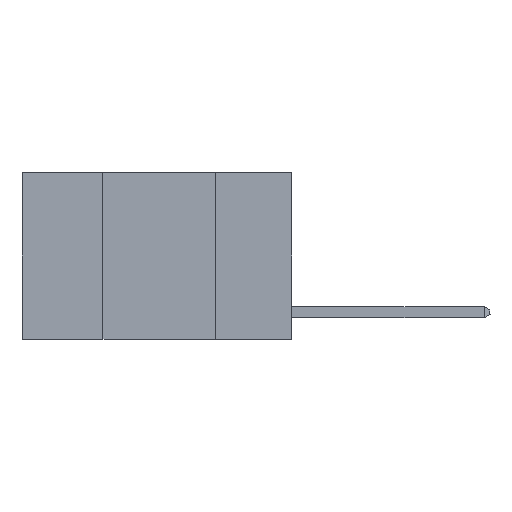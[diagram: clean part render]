
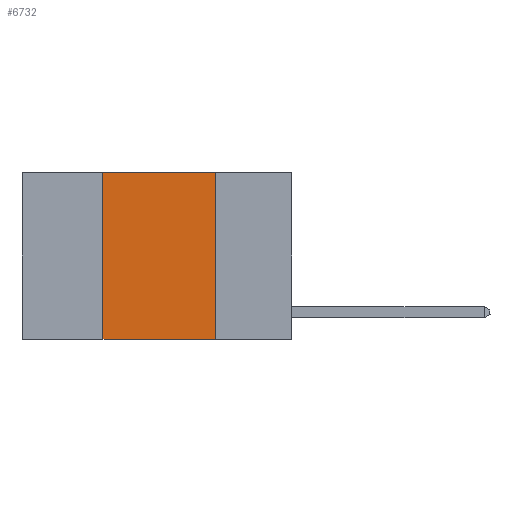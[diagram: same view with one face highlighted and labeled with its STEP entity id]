
A CAD part, left-side view. The second image highlights one B-rep face of the part: STEP entity #6732.
In plain terms, the highlighted planar face has unit normal (-1, 0, 0).
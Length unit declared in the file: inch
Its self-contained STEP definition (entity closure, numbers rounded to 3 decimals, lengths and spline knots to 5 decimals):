
#153 = EDGE_CURVE ( 'NONE', #2422, #431, #4611, .T. ) ;
#431 = VERTEX_POINT ( 'NONE', #10869 ) ;
#643 = VECTOR ( 'NONE', #11021, 39.37008 ) ;
#1158 = LINE ( 'NONE', #13587, #16704 ) ;
#1217 = CARTESIAN_POINT ( 'NONE',  ( 0., 0.42, 0. ) ) ;
#2249 = VECTOR ( 'NONE', #3580, 39.37008 ) ;
#2422 = VERTEX_POINT ( 'NONE', #1217 ) ;
#2770 = EDGE_CURVE ( 'NONE', #431, #12610, #14227, .T. ) ;
#3580 = DIRECTION ( 'NONE',  ( 0., 0., -1. ) ) ;
#3591 = ORIENTED_EDGE ( 'NONE', *, *, #153, .F. ) ;
#4251 = PLANE ( 'NONE',  #7774 ) ;
#4445 = LINE ( 'NONE', #16420, #9367 ) ;
#4611 = LINE ( 'NONE', #10774, #643 ) ;
#4911 = FACE_OUTER_BOUND ( 'NONE', #5931, .T. ) ;
#5931 = EDGE_LOOP ( 'NONE', ( #18127, #3591, #16023, #18744 ) ) ;
#6323 = EDGE_CURVE ( 'NONE', #6555, #2422, #1158, .T. ) ;
#6555 = VERTEX_POINT ( 'NONE', #15496 ) ;
#6732 = ADVANCED_FACE ( 'NONE', ( #4911 ), #4251, .F. ) ;
#7422 = DIRECTION ( 'NONE',  ( 1., 0., 0. ) ) ;
#7774 = AXIS2_PLACEMENT_3D ( 'NONE', #13431, #7422, #8637 ) ;
#8637 = DIRECTION ( 'NONE',  ( 0., 0., -1. ) ) ;
#9367 = VECTOR ( 'NONE', #10347, 39.37008 ) ;
#9798 = CARTESIAN_POINT ( 'NONE',  ( 0., 0.17, 0. ) ) ;
#10347 = DIRECTION ( 'NONE',  ( 0., -1., 0. ) ) ;
#10774 = CARTESIAN_POINT ( 'NONE',  ( 0., 0.6, 0. ) ) ;
#10869 = CARTESIAN_POINT ( 'NONE',  ( 0., 0.17, 0. ) ) ;
#11021 = DIRECTION ( 'NONE',  ( 0., -1., 0. ) ) ;
#12610 = VERTEX_POINT ( 'NONE', #18444 ) ;
#13431 = CARTESIAN_POINT ( 'NONE',  ( 0., 0.6, 0. ) ) ;
#13587 = CARTESIAN_POINT ( 'NONE',  ( 0., 0.42, 0. ) ) ;
#13664 = EDGE_CURVE ( 'NONE', #6555, #12610, #4445, .T. ) ;
#14227 = LINE ( 'NONE', #9798, #2249 ) ;
#15496 = CARTESIAN_POINT ( 'NONE',  ( 0., 0.42, -0.37 ) ) ;
#16023 = ORIENTED_EDGE ( 'NONE', *, *, #6323, .F. ) ;
#16390 = DIRECTION ( 'NONE',  ( 0., 0., 1. ) ) ;
#16420 = CARTESIAN_POINT ( 'NONE',  ( 0., 0.6, -0.37 ) ) ;
#16704 = VECTOR ( 'NONE', #16390, 39.37008 ) ;
#18127 = ORIENTED_EDGE ( 'NONE', *, *, #2770, .F. ) ;
#18444 = CARTESIAN_POINT ( 'NONE',  ( 0., 0.17, -0.37 ) ) ;
#18744 = ORIENTED_EDGE ( 'NONE', *, *, #13664, .T. ) ;
